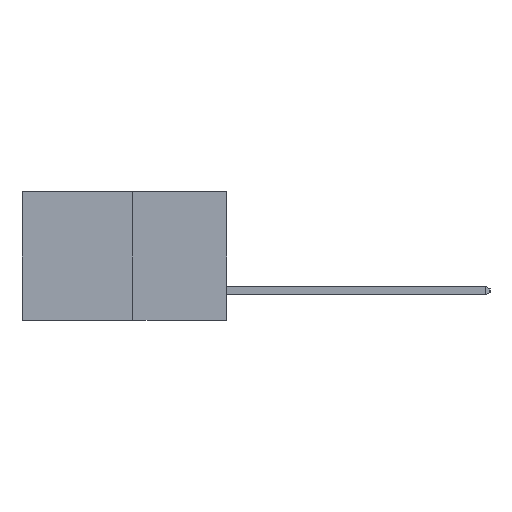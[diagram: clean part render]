
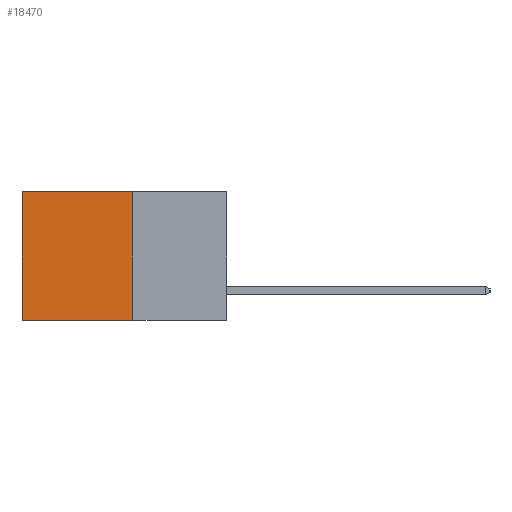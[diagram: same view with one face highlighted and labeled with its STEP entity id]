
A CAD part, left-side view. The second image highlights one B-rep face of the part: STEP entity #18470.
In plain terms, the highlighted planar face has unit normal (-1, 0, 0).
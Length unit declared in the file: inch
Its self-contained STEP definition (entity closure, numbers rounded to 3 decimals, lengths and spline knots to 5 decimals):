
#150 = DIRECTION ( 'NONE',  ( 0., 0., -1. ) ) ;
#283 = VECTOR ( 'NONE', #2046, 39.37008 ) ;
#319 = CARTESIAN_POINT ( 'NONE',  ( 0.277, 0.27, -0.37 ) ) ;
#983 = CARTESIAN_POINT ( 'NONE',  ( 0.277, 0.27, -0.37 ) ) ;
#1359 = LINE ( 'NONE', #319, #283 ) ;
#1694 = CARTESIAN_POINT ( 'NONE',  ( 0.277, 0.27, 0. ) ) ;
#1895 = EDGE_LOOP ( 'NONE', ( #11441, #4377, #19223, #11707 ) ) ;
#2046 = DIRECTION ( 'NONE',  ( 0., 0., -1. ) ) ;
#2738 = PLANE ( 'NONE',  #9070 ) ;
#2916 = VERTEX_POINT ( 'NONE', #7994 ) ;
#3756 = LINE ( 'NONE', #1694, #7569 ) ;
#4333 = LINE ( 'NONE', #13153, #20404 ) ;
#4371 = DIRECTION ( 'NONE',  ( 1., 0., 0. ) ) ;
#4377 = ORIENTED_EDGE ( 'NONE', *, *, #8554, .F. ) ;
#6894 = DIRECTION ( 'NONE',  ( 0., 1., 0. ) ) ;
#7005 = FACE_OUTER_BOUND ( 'NONE', #1895, .T. ) ;
#7569 = VECTOR ( 'NONE', #12996, 39.37008 ) ;
#7994 = CARTESIAN_POINT ( 'NONE',  ( 0.277, 0.59, 0. ) ) ;
#8554 = EDGE_CURVE ( 'NONE', #11855, #18421, #12814, .T. ) ;
#8565 = VECTOR ( 'NONE', #6894, 39.37008 ) ;
#9070 = AXIS2_PLACEMENT_3D ( 'NONE', #12386, #4371, #15597 ) ;
#11441 = ORIENTED_EDGE ( 'NONE', *, *, #20199, .T. ) ;
#11707 = ORIENTED_EDGE ( 'NONE', *, *, #17569, .T. ) ;
#11855 = VERTEX_POINT ( 'NONE', #983 ) ;
#12386 = CARTESIAN_POINT ( 'NONE',  ( 0.277, 0.27, -0.37 ) ) ;
#12814 = LINE ( 'NONE', #14938, #8565 ) ;
#12996 = DIRECTION ( 'NONE',  ( 0., 1., 0. ) ) ;
#13153 = CARTESIAN_POINT ( 'NONE',  ( 0.277, 0.59, -0.37 ) ) ;
#14938 = CARTESIAN_POINT ( 'NONE',  ( 0.277, 0.27, -0.37 ) ) ;
#15597 = DIRECTION ( 'NONE',  ( 0., 0., -1. ) ) ;
#17569 = EDGE_CURVE ( 'NONE', #19175, #2916, #3756, .T. ) ;
#18383 = EDGE_CURVE ( 'NONE', #19175, #11855, #1359, .T. ) ;
#18421 = VERTEX_POINT ( 'NONE', #18729 ) ;
#18470 = ADVANCED_FACE ( 'NONE', ( #7005 ), #2738, .F. ) ;
#18729 = CARTESIAN_POINT ( 'NONE',  ( 0.277, 0.59, -0.37 ) ) ;
#19175 = VERTEX_POINT ( 'NONE', #20831 ) ;
#19223 = ORIENTED_EDGE ( 'NONE', *, *, #18383, .F. ) ;
#20199 = EDGE_CURVE ( 'NONE', #2916, #18421, #4333, .T. ) ;
#20404 = VECTOR ( 'NONE', #150, 39.37008 ) ;
#20831 = CARTESIAN_POINT ( 'NONE',  ( 0.277, 0.27, 0. ) ) ;
